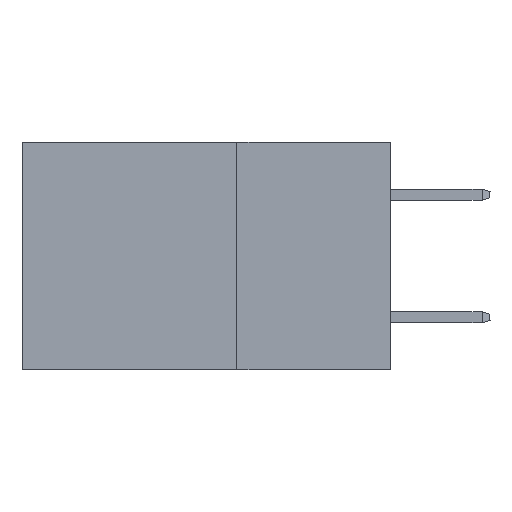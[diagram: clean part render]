
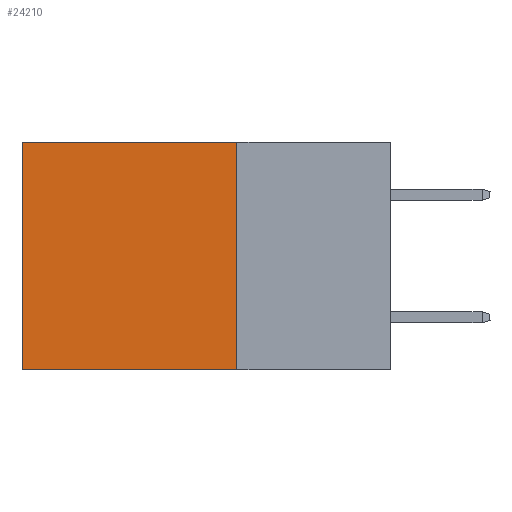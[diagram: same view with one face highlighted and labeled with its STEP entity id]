
A CAD part, left-side view. The second image highlights one B-rep face of the part: STEP entity #24210.
In plain terms, the highlighted planar face has unit normal (-1, 0, 0).
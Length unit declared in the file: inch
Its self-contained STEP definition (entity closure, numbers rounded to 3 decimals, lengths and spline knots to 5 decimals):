
#47 = VERTEX_POINT ( 'NONE', #6472 ) ;
#2037 = ORIENTED_EDGE ( 'NONE', *, *, #21408, .T. ) ;
#3258 = VECTOR ( 'NONE', #13946, 39.37008 ) ;
#3392 = CARTESIAN_POINT ( 'NONE',  ( 0.2875, 0.6, -0.37 ) ) ;
#3893 = DIRECTION ( 'NONE',  ( 0., 1., 0. ) ) ;
#4348 = CARTESIAN_POINT ( 'NONE',  ( 0.2875, 0.25, 0. ) ) ;
#5523 = VECTOR ( 'NONE', #17984, 39.37008 ) ;
#6327 = DIRECTION ( 'NONE',  ( 0., 0., -1. ) ) ;
#6472 = CARTESIAN_POINT ( 'NONE',  ( 0.2875, 0.25, -0.37 ) ) ;
#6618 = CARTESIAN_POINT ( 'NONE',  ( 0.2875, 0.25, 0. ) ) ;
#8248 = LINE ( 'NONE', #33494, #21331 ) ;
#8641 = AXIS2_PLACEMENT_3D ( 'NONE', #6618, #20075, #33683 ) ;
#8687 = EDGE_CURVE ( 'NONE', #11403, #16166, #12232, .T. ) ;
#9829 = CARTESIAN_POINT ( 'NONE',  ( 0.2875, 0.6, 0. ) ) ;
#11403 = VERTEX_POINT ( 'NONE', #4348 ) ;
#12232 = LINE ( 'NONE', #18452, #5523 ) ;
#13946 = DIRECTION ( 'NONE',  ( 0., 0., -1. ) ) ;
#14740 = PLANE ( 'NONE',  #8641 ) ;
#16166 = VERTEX_POINT ( 'NONE', #9829 ) ;
#17984 = DIRECTION ( 'NONE',  ( 0., 1., 0. ) ) ;
#18452 = CARTESIAN_POINT ( 'NONE',  ( 0.2875, 0.25, 0. ) ) ;
#19827 = CARTESIAN_POINT ( 'NONE',  ( 0.2875, 0.25, -0.37 ) ) ;
#20075 = DIRECTION ( 'NONE',  ( 1., 0., 0. ) ) ;
#20325 = EDGE_CURVE ( 'NONE', #47, #26108, #32947, .T. ) ;
#20883 = ORIENTED_EDGE ( 'NONE', *, *, #20325, .F. ) ;
#21125 = ORIENTED_EDGE ( 'NONE', *, *, #33446, .F. ) ;
#21331 = VECTOR ( 'NONE', #6327, 39.37008 ) ;
#21408 = EDGE_CURVE ( 'NONE', #16166, #26108, #26483, .T. ) ;
#23632 = VECTOR ( 'NONE', #3893, 39.37008 ) ;
#24210 = ADVANCED_FACE ( 'NONE', ( #27597 ), #14740, .F. ) ;
#26108 = VERTEX_POINT ( 'NONE', #3392 ) ;
#26157 = EDGE_LOOP ( 'NONE', ( #2037, #20883, #21125, #26270 ) ) ;
#26270 = ORIENTED_EDGE ( 'NONE', *, *, #8687, .T. ) ;
#26483 = LINE ( 'NONE', #29773, #3258 ) ;
#27597 = FACE_OUTER_BOUND ( 'NONE', #26157, .T. ) ;
#29773 = CARTESIAN_POINT ( 'NONE',  ( 0.2875, 0.6, 0. ) ) ;
#32947 = LINE ( 'NONE', #19827, #23632 ) ;
#33446 = EDGE_CURVE ( 'NONE', #11403, #47, #8248, .T. ) ;
#33494 = CARTESIAN_POINT ( 'NONE',  ( 0.2875, 0.25, 0. ) ) ;
#33683 = DIRECTION ( 'NONE',  ( 0., 0., -1. ) ) ;
